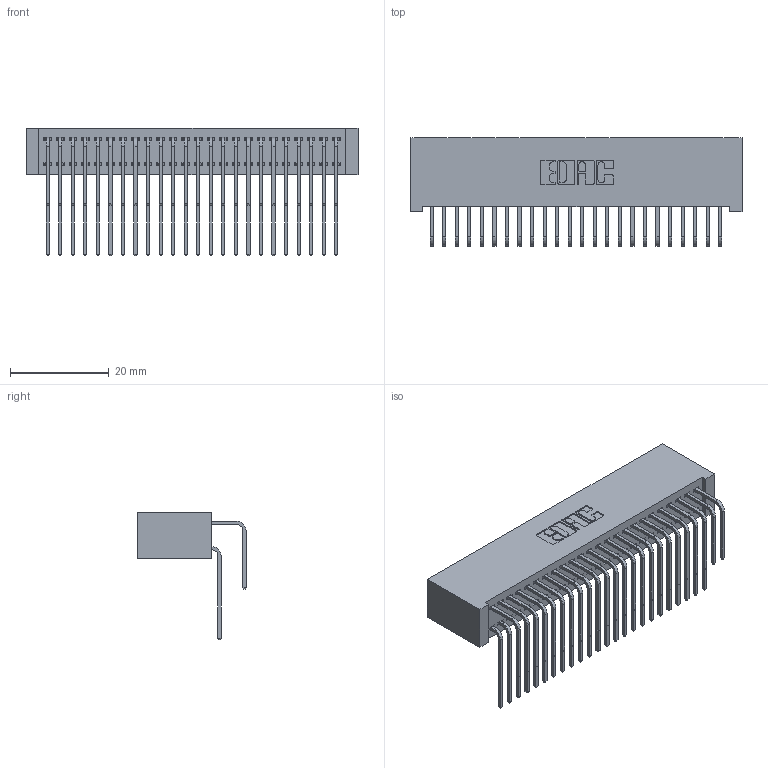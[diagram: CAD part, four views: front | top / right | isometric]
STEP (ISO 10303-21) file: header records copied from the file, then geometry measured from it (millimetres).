
FILE_DESCRIPTION (( 'STEP AP203' ), '1' );
FILE_NAME ('392-048-558-201.STEP', '2019-10-08T01:29:11', ( '' ), ( '' ), 'SwSTEP 2.0', 'SolidWorks 2016', '' );
FILE_SCHEMA (( 'CONFIG_CONTROL_DESIGN' ));
Length unit declared in the file: inch
Products named in the file (4): 392-048-558-201; 342 Part_Lugless; 345-292-001_558 559 Tail - 1; 345-292-001_558 Tail - 2
Assembly tree (49 placements, depth 2):
  392-048-558-201
    342 Part_Lugless
    345-292-001_558 559 Tail - 1  x24
    345-292-001_558 Tail - 2  x24
Bounding box: 67.21 x 21.91 x 25.78 mm (x, y, z)
Volume: 6669.9 mm3; surface area: 12112.2 mm2
Topology: 49 solids, 49 shells, 2694 faces, 8003 edges, 5270 vertices
Faces by surface type: plane 1886, cylinder 808
Entity records: 19143 total; most frequent: CARTESIAN_POINT 3241, ORIENTED_EDGE 3126, DIRECTION 2775, EDGE_CURVE 1563, VECTOR 1403, LINE 1403, VERTEX_POINT 1038, AXIS2_PLACEMENT_3D 686
